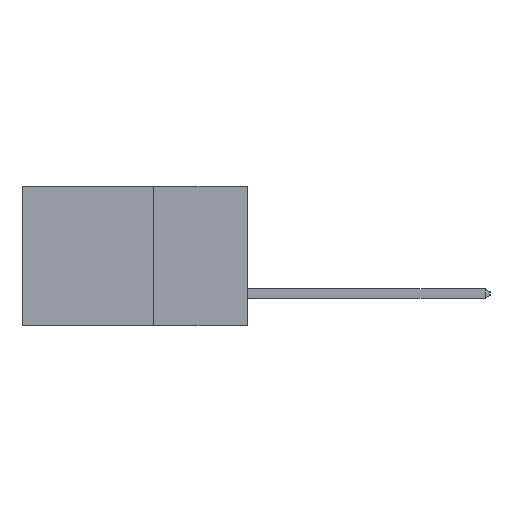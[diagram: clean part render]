
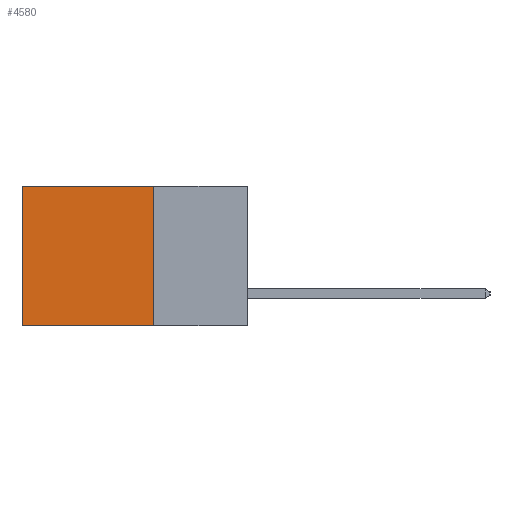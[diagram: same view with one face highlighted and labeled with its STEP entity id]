
A CAD part, left-side view. The second image highlights one B-rep face of the part: STEP entity #4580.
In plain terms, the highlighted planar face has unit normal (-1, 0, 0).
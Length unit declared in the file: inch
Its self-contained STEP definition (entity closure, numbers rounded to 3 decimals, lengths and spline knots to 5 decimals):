
#1853 = DIRECTION ( 'NONE',  ( 0., 1., 0. ) ) ;
#2347 = ORIENTED_EDGE ( 'NONE', *, *, #22411, .T. ) ;
#4266 = EDGE_CURVE ( 'NONE', #20922, #20356, #6679, .T. ) ;
#4391 = CARTESIAN_POINT ( 'NONE',  ( 0.298, 0.25, 0. ) ) ;
#4580 = ADVANCED_FACE ( 'NONE', ( #7849 ), #15829, .F. ) ;
#5350 = DIRECTION ( 'NONE',  ( 1., 0., 0. ) ) ;
#6262 = CARTESIAN_POINT ( 'NONE',  ( 0.298, 0.25, 0. ) ) ;
#6529 = VERTEX_POINT ( 'NONE', #10656 ) ;
#6679 = LINE ( 'NONE', #4391, #20598 ) ;
#7849 = FACE_OUTER_BOUND ( 'NONE', #10632, .T. ) ;
#8210 = VECTOR ( 'NONE', #16735, 39.37008 ) ;
#8225 = DIRECTION ( 'NONE',  ( 0., 0., -1. ) ) ;
#8804 = CARTESIAN_POINT ( 'NONE',  ( 0.298, 0.25, 0. ) ) ;
#8824 = CARTESIAN_POINT ( 'NONE',  ( 0.298, 0.25, -0.37 ) ) ;
#9053 = VECTOR ( 'NONE', #8225, 39.37008 ) ;
#9273 = VECTOR ( 'NONE', #1853, 39.37008 ) ;
#10632 = EDGE_LOOP ( 'NONE', ( #2347, #20405, #13766, #22203 ) ) ;
#10656 = CARTESIAN_POINT ( 'NONE',  ( 0.298, 0.6, 0. ) ) ;
#10773 = VERTEX_POINT ( 'NONE', #19812 ) ;
#13234 = DIRECTION ( 'NONE',  ( 0., 0., -1. ) ) ;
#13766 = ORIENTED_EDGE ( 'NONE', *, *, #4266, .F. ) ;
#13919 = LINE ( 'NONE', #18488, #8210 ) ;
#14227 = LINE ( 'NONE', #22161, #9053 ) ;
#15559 = LINE ( 'NONE', #8824, #9273 ) ;
#15829 = PLANE ( 'NONE',  #20810 ) ;
#16669 = EDGE_CURVE ( 'NONE', #20356, #10773, #15559, .T. ) ;
#16735 = DIRECTION ( 'NONE',  ( 0., 1., 0. ) ) ;
#16784 = CARTESIAN_POINT ( 'NONE',  ( 0.298, 0.25, -0.37 ) ) ;
#17623 = DIRECTION ( 'NONE',  ( 0., 0., -1. ) ) ;
#18488 = CARTESIAN_POINT ( 'NONE',  ( 0.298, 0.25, 0. ) ) ;
#19812 = CARTESIAN_POINT ( 'NONE',  ( 0.298, 0.6, -0.37 ) ) ;
#20356 = VERTEX_POINT ( 'NONE', #16784 ) ;
#20405 = ORIENTED_EDGE ( 'NONE', *, *, #16669, .F. ) ;
#20598 = VECTOR ( 'NONE', #13234, 39.37008 ) ;
#20810 = AXIS2_PLACEMENT_3D ( 'NONE', #8804, #5350, #17623 ) ;
#20922 = VERTEX_POINT ( 'NONE', #6262 ) ;
#21551 = EDGE_CURVE ( 'NONE', #20922, #6529, #13919, .T. ) ;
#22161 = CARTESIAN_POINT ( 'NONE',  ( 0.298, 0.6, 0. ) ) ;
#22203 = ORIENTED_EDGE ( 'NONE', *, *, #21551, .T. ) ;
#22411 = EDGE_CURVE ( 'NONE', #6529, #10773, #14227, .T. ) ;
